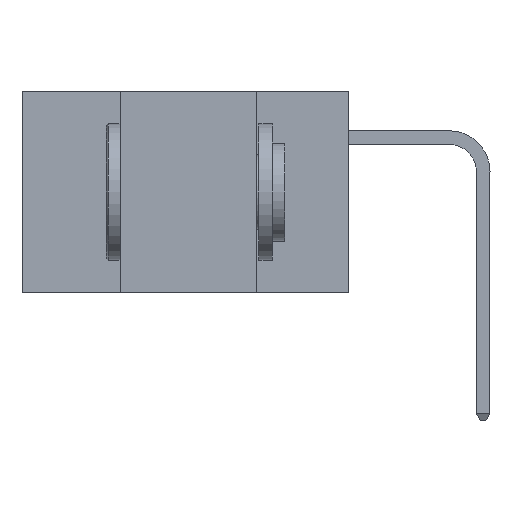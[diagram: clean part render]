
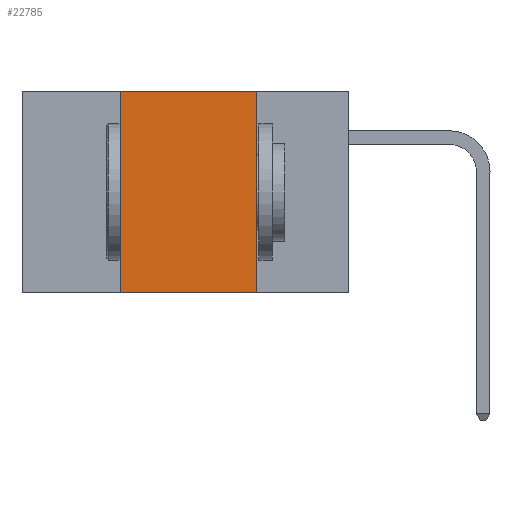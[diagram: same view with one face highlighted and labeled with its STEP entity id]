
A CAD part, left-side view. The second image highlights one B-rep face of the part: STEP entity #22785.
In plain terms, the highlighted planar face has unit normal (-1, 0, 0).
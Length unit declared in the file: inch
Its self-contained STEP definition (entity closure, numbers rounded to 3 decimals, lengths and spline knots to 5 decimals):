
#1375 = DIRECTION ( 'NONE',  ( 0., 0., -1. ) ) ;
#1691 = CARTESIAN_POINT ( 'NONE',  ( 0., 0.6, -0.37 ) ) ;
#2358 = CARTESIAN_POINT ( 'NONE',  ( 0., 0.42, 0. ) ) ;
#2421 = EDGE_CURVE ( 'NONE', #8485, #2775, #11526, .T. ) ;
#2775 = VERTEX_POINT ( 'NONE', #6523 ) ;
#5887 = EDGE_CURVE ( 'NONE', #27115, #2775, #35002, .T. ) ;
#5900 = EDGE_LOOP ( 'NONE', ( #7560, #6130, #35278, #38221 ) ) ;
#6049 = VECTOR ( 'NONE', #30038, 39.37008 ) ;
#6130 = ORIENTED_EDGE ( 'NONE', *, *, #36284, .F. ) ;
#6523 = CARTESIAN_POINT ( 'NONE',  ( 0., 0.17, -0.37 ) ) ;
#7560 = ORIENTED_EDGE ( 'NONE', *, *, #5887, .F. ) ;
#8485 = VERTEX_POINT ( 'NONE', #10819 ) ;
#10819 = CARTESIAN_POINT ( 'NONE',  ( 0., 0.42, -0.37 ) ) ;
#10854 = DIRECTION ( 'NONE',  ( 0., -1., 0. ) ) ;
#11526 = LINE ( 'NONE', #1691, #29234 ) ;
#12865 = VECTOR ( 'NONE', #13606, 39.37008 ) ;
#13606 = DIRECTION ( 'NONE',  ( 0., 0., 1. ) ) ;
#15976 = PLANE ( 'NONE',  #22461 ) ;
#19000 = DIRECTION ( 'NONE',  ( 1., 0., 0. ) ) ;
#19401 = CARTESIAN_POINT ( 'NONE',  ( 0., 0.17, 0. ) ) ;
#21468 = LINE ( 'NONE', #25733, #27052 ) ;
#22461 = AXIS2_PLACEMENT_3D ( 'NONE', #30964, #19000, #1375 ) ;
#22593 = VERTEX_POINT ( 'NONE', #2358 ) ;
#22735 = CARTESIAN_POINT ( 'NONE',  ( 0., 0.42, 0. ) ) ;
#22785 = ADVANCED_FACE ( 'NONE', ( #33063 ), #15976, .F. ) ;
#23824 = CARTESIAN_POINT ( 'NONE',  ( 0., 0.17, 0. ) ) ;
#24346 = EDGE_CURVE ( 'NONE', #8485, #22593, #33864, .T. ) ;
#25471 = DIRECTION ( 'NONE',  ( 0., -1., 0. ) ) ;
#25733 = CARTESIAN_POINT ( 'NONE',  ( 0., 0.6, 0. ) ) ;
#27052 = VECTOR ( 'NONE', #25471, 39.37008 ) ;
#27115 = VERTEX_POINT ( 'NONE', #19401 ) ;
#29234 = VECTOR ( 'NONE', #10854, 39.37008 ) ;
#30038 = DIRECTION ( 'NONE',  ( 0., 0., -1. ) ) ;
#30964 = CARTESIAN_POINT ( 'NONE',  ( 0., 0.6, 0. ) ) ;
#33063 = FACE_OUTER_BOUND ( 'NONE', #5900, .T. ) ;
#33864 = LINE ( 'NONE', #22735, #12865 ) ;
#35002 = LINE ( 'NONE', #23824, #6049 ) ;
#35278 = ORIENTED_EDGE ( 'NONE', *, *, #24346, .F. ) ;
#36284 = EDGE_CURVE ( 'NONE', #22593, #27115, #21468, .T. ) ;
#38221 = ORIENTED_EDGE ( 'NONE', *, *, #2421, .T. ) ;
